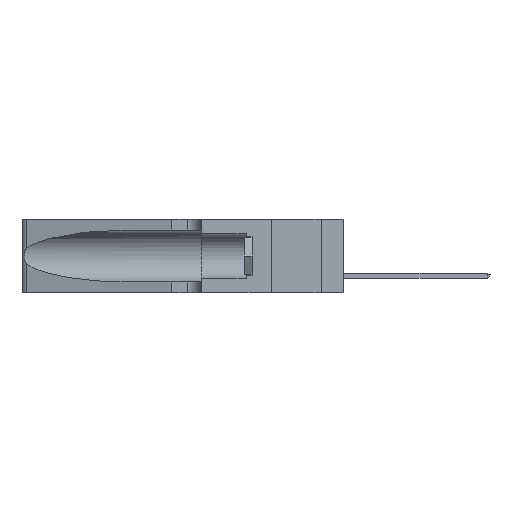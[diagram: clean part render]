
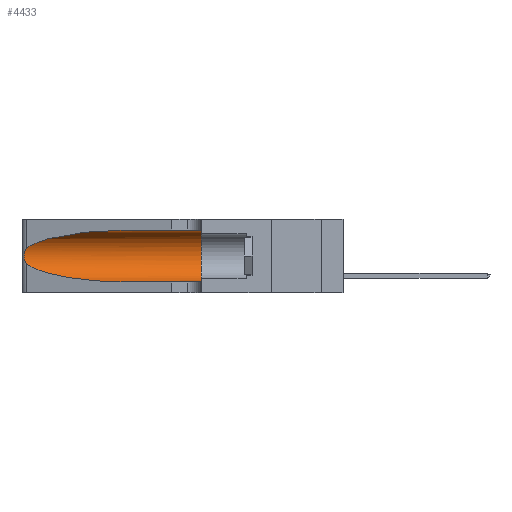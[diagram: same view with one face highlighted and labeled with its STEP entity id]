
A CAD part, left-side view. The second image highlights one B-rep face of the part: STEP entity #4433.
In plain terms, the highlighted cylindrical face has radius 3.308 mm (diameter 6.617 mm), a partial arc.
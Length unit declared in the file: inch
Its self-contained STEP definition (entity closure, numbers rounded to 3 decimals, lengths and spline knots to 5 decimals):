
#231 =( BOUNDED_CURVE ( )  B_SPLINE_CURVE ( 3, ( #21556, #17244, #8512, #21371 ),
 .UNSPECIFIED., .F., .F. ) 
 B_SPLINE_CURVE_WITH_KNOTS ( ( 4, 4 ),
 ( 3.44316, 4.71239 ),
 .UNSPECIFIED. ) 
 CURVE ( )  GEOMETRIC_REPRESENTATION_ITEM ( )  RATIONAL_B_SPLINE_CURVE ( ( 1., 0.87, 0.87, 1. ) ) 
 REPRESENTATION_ITEM ( '' )  );
#1041 = CARTESIAN_POINT ( 'NONE',  ( 0.25487, 1.22718, 0.22369 ) ) ;
#1173 = CARTESIAN_POINT ( 'NONE',  ( 0.26018, 1.23835, 0.19895 ) ) ;
#2096 = VERTEX_POINT ( 'NONE', #13111 ) ;
#3079 = DIRECTION ( 'NONE',  ( 0., -1., 0. ) ) ;
#3313 = CARTESIAN_POINT ( 'NONE',  ( 0.25487, 1.22718, 0.22369 ) ) ;
#3479 = DIRECTION ( 'NONE',  ( 0., -1., 0. ) ) ;
#3505 = CARTESIAN_POINT ( 'NONE',  ( 0.26075, 1.23896, 0.178 ) ) ;
#3946 = AXIS2_PLACEMENT_3D ( 'NONE', #11805, #3079, #7462 ) ;
#4299 = ORIENTED_EDGE ( 'NONE', *, *, #18852, .F. ) ;
#4433 = ADVANCED_FACE ( 'NONE', ( #7272 ), #25486, .F. ) ;
#5333 = B_SPLINE_CURVE_WITH_KNOTS ( 'NONE', 3,
 ( #3313, #9996, #25046, #12033, #5394, #1173, #20913, #3505, #11936, #25345, #18828, #5687, #10089, #12318 ),
 .UNSPECIFIED., .F., .F.,
 ( 4, 2, 2, 2, 2, 2, 4 ),
 ( 0., 0.00027, 0.00053, 0.00107, 0.0016, 0.00187, 0.00214 ),
 .UNSPECIFIED. ) ;
#5394 = CARTESIAN_POINT ( 'NONE',  ( 0.25854, 1.2359, 0.20912 ) ) ;
#5661 = CARTESIAN_POINT ( 'NONE',  ( 0.1305, 1.61858, 0.31525 ) ) ;
#5687 = CARTESIAN_POINT ( 'NONE',  ( 0.25639, 1.23186, 0.15144 ) ) ;
#6895 = ORIENTED_EDGE ( 'NONE', *, *, #22666, .T. ) ;
#6993 = ORIENTED_EDGE ( 'NONE', *, *, #12316, .T. ) ;
#7272 = FACE_OUTER_BOUND ( 'NONE', #25899, .T. ) ;
#7462 = DIRECTION ( 'NONE',  ( 0., 0., -1. ) ) ;
#8163 = DIRECTION ( 'NONE',  ( 0., 1., 0. ) ) ;
#8512 = CARTESIAN_POINT ( 'NONE',  ( 0.18966, 0.96281, 0.05475 ) ) ;
#9657 = VERTEX_POINT ( 'NONE', #19348 ) ;
#9996 = CARTESIAN_POINT ( 'NONE',  ( 0.25555, 1.22994, 0.2215 ) ) ;
#10089 = CARTESIAN_POINT ( 'NONE',  ( 0.25555, 1.22993, 0.14849 ) ) ;
#10742 = VECTOR ( 'NONE', #3479, 39.37008 ) ;
#11805 = CARTESIAN_POINT ( 'NONE',  ( 0.1305, 1.61858, 0.185 ) ) ;
#11936 = CARTESIAN_POINT ( 'NONE',  ( 0.26017, 1.23833, 0.17102 ) ) ;
#12033 = CARTESIAN_POINT ( 'NONE',  ( 0.25787, 1.23484, 0.2124 ) ) ;
#12316 = EDGE_CURVE ( 'NONE', #18357, #20393, #19402, .T. ) ;
#12318 = CARTESIAN_POINT ( 'NONE',  ( 0.25487, 1.22718, 0.14631 ) ) ;
#12482 = CARTESIAN_POINT ( 'NONE',  ( 0.25487, 1.22718, 0.14631 ) ) ;
#13111 = CARTESIAN_POINT ( 'NONE',  ( 0.1305, 0.35, 0.05475 ) ) ;
#13950 = VERTEX_POINT ( 'NONE', #12482 ) ;
#16495 = CARTESIAN_POINT ( 'NONE',  ( 0.18966, 0.96281, 0.31525 ) ) ;
#16804 = CARTESIAN_POINT ( 'NONE',  ( 0.1305, 0.35, 0.185 ) ) ;
#17106 = CARTESIAN_POINT ( 'NONE',  ( 0.1305, 0.72297, 0.05475 ) ) ;
#17153 = LINE ( 'NONE', #24682, #25374 ) ;
#17244 = CARTESIAN_POINT ( 'NONE',  ( 0.2373, 1.15595, 0.08982 ) ) ;
#18357 = VERTEX_POINT ( 'NONE', #22873 ) ;
#18407 = CARTESIAN_POINT ( 'NONE',  ( 0.2373, 1.15595, 0.28018 ) ) ;
#18475 = CIRCLE ( 'NONE', #23749, 0.13025 ) ;
#18828 = CARTESIAN_POINT ( 'NONE',  ( 0.25789, 1.23486, 0.15765 ) ) ;
#18852 = EDGE_CURVE ( 'NONE', #18357, #9657, #22072, .T. ) ;
#19348 = CARTESIAN_POINT ( 'NONE',  ( 0.1305, 0.35, 0.31525 ) ) ;
#19402 =( BOUNDED_CURVE ( )  B_SPLINE_CURVE ( 3, ( #22900, #16495, #18407, #1041 ),
 .UNSPECIFIED., .F., .T. ) 
 B_SPLINE_CURVE_WITH_KNOTS ( ( 4, 4 ),
 ( 1.5708, 2.84003 ),
 .UNSPECIFIED. ) 
 CURVE ( )  GEOMETRIC_REPRESENTATION_ITEM ( )  RATIONAL_B_SPLINE_CURVE ( ( 1., 0.87, 0.87, 1. ) ) 
 REPRESENTATION_ITEM ( '' )  );
#19730 = ORIENTED_EDGE ( 'NONE', *, *, #20507, .T. ) ;
#19798 = EDGE_CURVE ( 'NONE', #20393, #13950, #5333, .T. ) ;
#20393 = VERTEX_POINT ( 'NONE', #23205 ) ;
#20507 = EDGE_CURVE ( 'NONE', #13950, #26738, #231, .T. ) ;
#20913 = CARTESIAN_POINT ( 'NONE',  ( 0.26075, 1.23896, 0.19203 ) ) ;
#21098 = DIRECTION ( 'NONE',  ( 0., 0., 1. ) ) ;
#21371 = CARTESIAN_POINT ( 'NONE',  ( 0.1305, 0.72297, 0.05475 ) ) ;
#21439 = ORIENTED_EDGE ( 'NONE', *, *, #23399, .F. ) ;
#21556 = CARTESIAN_POINT ( 'NONE',  ( 0.25487, 1.22718, 0.14631 ) ) ;
#22072 = LINE ( 'NONE', #5661, #10742 ) ;
#22666 = EDGE_CURVE ( 'NONE', #26738, #2096, #17153, .T. ) ;
#22873 = CARTESIAN_POINT ( 'NONE',  ( 0.1305, 0.72297, 0.31525 ) ) ;
#22900 = CARTESIAN_POINT ( 'NONE',  ( 0.1305, 0.72297, 0.31525 ) ) ;
#23205 = CARTESIAN_POINT ( 'NONE',  ( 0.25487, 1.22718, 0.22369 ) ) ;
#23399 = EDGE_CURVE ( 'NONE', #9657, #2096, #18475, .T. ) ;
#23749 = AXIS2_PLACEMENT_3D ( 'NONE', #16804, #8163, #21098 ) ;
#24682 = CARTESIAN_POINT ( 'NONE',  ( 0.1305, 1.61858, 0.05475 ) ) ;
#25046 = CARTESIAN_POINT ( 'NONE',  ( 0.25639, 1.23184, 0.21858 ) ) ;
#25345 = CARTESIAN_POINT ( 'NONE',  ( 0.25856, 1.23593, 0.16098 ) ) ;
#25374 = VECTOR ( 'NONE', #26773, 39.37008 ) ;
#25486 = CYLINDRICAL_SURFACE ( 'NONE', #3946, 0.13025 ) ;
#25899 = EDGE_LOOP ( 'NONE', ( #6993, #26442, #19730, #6895, #21439, #4299 ) ) ;
#26442 = ORIENTED_EDGE ( 'NONE', *, *, #19798, .T. ) ;
#26738 = VERTEX_POINT ( 'NONE', #17106 ) ;
#26773 = DIRECTION ( 'NONE',  ( 0., -1., 0. ) ) ;
